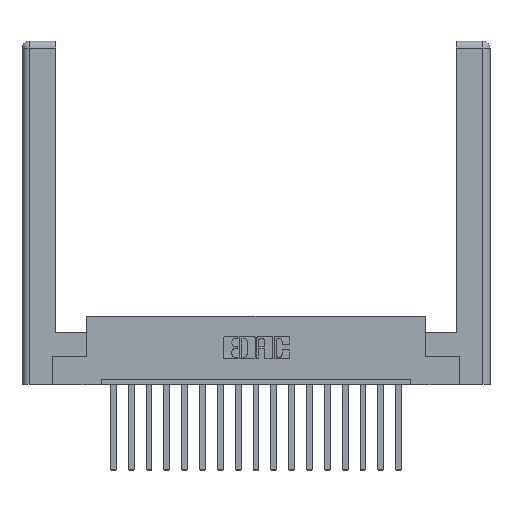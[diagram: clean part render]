
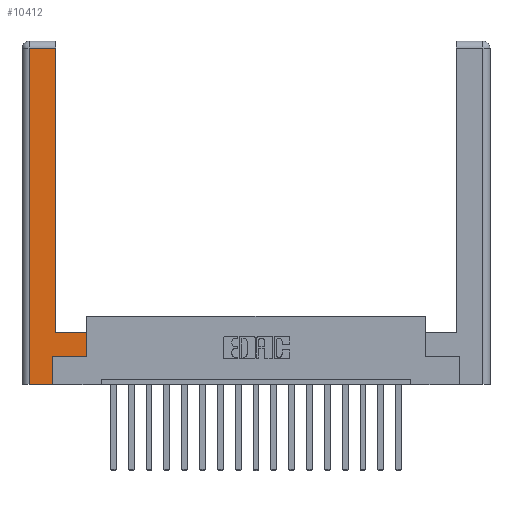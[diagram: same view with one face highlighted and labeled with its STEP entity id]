
A CAD part, top view. The second image highlights one B-rep face of the part: STEP entity #10412.
In plain terms, the highlighted planar face has unit normal (0, 0, 1).
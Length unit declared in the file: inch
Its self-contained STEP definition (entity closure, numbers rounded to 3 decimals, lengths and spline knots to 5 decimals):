
#91 = ORIENTED_EDGE ( 'NONE', *, *, #14278, .T. ) ;
#585 = VECTOR ( 'NONE', #4979, 39.37008 ) ;
#655 = CARTESIAN_POINT ( 'NONE',  ( 0.295, 0.45, 0. ) ) ;
#868 = VERTEX_POINT ( 'NONE', #13575 ) ;
#1252 = AXIS2_PLACEMENT_3D ( 'NONE', #9965, #9904, #9846 ) ;
#1298 = EDGE_CURVE ( 'NONE', #14913, #5578, #17673, .T. ) ;
#1403 = VECTOR ( 'NONE', #15407, 39.37008 ) ;
#1578 = CARTESIAN_POINT ( 'NONE',  ( 0.0615, 2.94, 0. ) ) ;
#1925 = VERTEX_POINT ( 'NONE', #12431 ) ;
#2137 = CARTESIAN_POINT ( 'NONE',  ( 0.0615, 2.94, 0. ) ) ;
#2154 = CARTESIAN_POINT ( 'NONE',  ( 0.565, 0.45, 0. ) ) ;
#2252 = ORIENTED_EDGE ( 'NONE', *, *, #13326, .T. ) ;
#2303 = DIRECTION ( 'NONE',  ( -1., 0., 0. ) ) ;
#2349 = VERTEX_POINT ( 'NONE', #655 ) ;
#2746 = DIRECTION ( 'NONE',  ( 1., 0., 0. ) ) ;
#3480 = VECTOR ( 'NONE', #2303, 39.37008 ) ;
#3620 = CARTESIAN_POINT ( 'NONE',  ( 0.0615, 0., 0. ) ) ;
#4251 = ORIENTED_EDGE ( 'NONE', *, *, #14342, .T. ) ;
#4393 = VECTOR ( 'NONE', #14295, 39.37008 ) ;
#4441 = EDGE_LOOP ( 'NONE', ( #16460, #12701, #6560, #2252, #91, #16508, #8641, #4251 ) ) ;
#4615 = LINE ( 'NONE', #1578, #4393 ) ;
#4620 = DIRECTION ( 'NONE',  ( 1., 0., 0. ) ) ;
#4720 = EDGE_CURVE ( 'NONE', #1925, #11762, #4615, .T. ) ;
#4979 = DIRECTION ( 'NONE',  ( 0., 1., 0. ) ) ;
#5578 = VERTEX_POINT ( 'NONE', #2154 ) ;
#5974 = CARTESIAN_POINT ( 'NONE',  ( 0.265, 0., 0. ) ) ;
#6349 = VERTEX_POINT ( 'NONE', #10061 ) ;
#6415 = VECTOR ( 'NONE', #16242, 39.37008 ) ;
#6509 = CARTESIAN_POINT ( 'NONE',  ( 0.295, 0.45, 0. ) ) ;
#6560 = ORIENTED_EDGE ( 'NONE', *, *, #11908, .T. ) ;
#6600 = EDGE_CURVE ( 'NONE', #2349, #1925, #16486, .T. ) ;
#6794 = LINE ( 'NONE', #13414, #585 ) ;
#6891 = CARTESIAN_POINT ( 'NONE',  ( 0.565, 0.245, 0. ) ) ;
#7680 = DIRECTION ( 'NONE',  ( 0., -1., 0. ) ) ;
#7972 = CARTESIAN_POINT ( 'NONE',  ( 0.565, 0.245, 0. ) ) ;
#8641 = ORIENTED_EDGE ( 'NONE', *, *, #1298, .T. ) ;
#8693 = PLANE ( 'NONE',  #1252 ) ;
#8758 = LINE ( 'NONE', #6509, #3480 ) ;
#8839 = VECTOR ( 'NONE', #7680, 39.37008 ) ;
#9343 = VERTEX_POINT ( 'NONE', #11339 ) ;
#9665 = VECTOR ( 'NONE', #2746, 39.37008 ) ;
#9846 = DIRECTION ( 'NONE',  ( -1., 0., 0. ) ) ;
#9904 = DIRECTION ( 'NONE',  ( 0., 0., -1. ) ) ;
#9965 = CARTESIAN_POINT ( 'NONE',  ( 0., 0., 0. ) ) ;
#10061 = CARTESIAN_POINT ( 'NONE',  ( 0.0615, 0., 0. ) ) ;
#10412 = ADVANCED_FACE ( 'NONE', ( #10854 ), #8693, .F. ) ;
#10854 = FACE_OUTER_BOUND ( 'NONE', #4441, .T. ) ;
#11169 = CARTESIAN_POINT ( 'NONE',  ( 0.295, 3., 0. ) ) ;
#11339 = CARTESIAN_POINT ( 'NONE',  ( 0.265, 0.245, 0. ) ) ;
#11762 = VERTEX_POINT ( 'NONE', #2137 ) ;
#11908 = EDGE_CURVE ( 'NONE', #11762, #6349, #16156, .T. ) ;
#12431 = CARTESIAN_POINT ( 'NONE',  ( 0.295, 2.94, 0. ) ) ;
#12701 = ORIENTED_EDGE ( 'NONE', *, *, #4720, .T. ) ;
#13185 = EDGE_CURVE ( 'NONE', #9343, #14913, #16769, .T. ) ;
#13326 = EDGE_CURVE ( 'NONE', #6349, #868, #14968, .T. ) ;
#13414 = CARTESIAN_POINT ( 'NONE',  ( 0.265, 0.245, 0. ) ) ;
#13575 = CARTESIAN_POINT ( 'NONE',  ( 0.265, 0., 0. ) ) ;
#14278 = EDGE_CURVE ( 'NONE', #868, #9343, #6794, .T. ) ;
#14295 = DIRECTION ( 'NONE',  ( -1., 0., 0. ) ) ;
#14342 = EDGE_CURVE ( 'NONE', #5578, #2349, #8758, .T. ) ;
#14913 = VERTEX_POINT ( 'NONE', #7972 ) ;
#14968 = LINE ( 'NONE', #5974, #18097 ) ;
#15407 = DIRECTION ( 'NONE',  ( 0., 1., 0. ) ) ;
#16156 = LINE ( 'NONE', #3620, #8839 ) ;
#16242 = DIRECTION ( 'NONE',  ( 0., 1., 0. ) ) ;
#16460 = ORIENTED_EDGE ( 'NONE', *, *, #6600, .T. ) ;
#16486 = LINE ( 'NONE', #11169, #1403 ) ;
#16508 = ORIENTED_EDGE ( 'NONE', *, *, #13185, .T. ) ;
#16769 = LINE ( 'NONE', #6891, #9665 ) ;
#17571 = CARTESIAN_POINT ( 'NONE',  ( 0.565, 0.45, 0. ) ) ;
#17673 = LINE ( 'NONE', #17571, #6415 ) ;
#18097 = VECTOR ( 'NONE', #4620, 39.37008 ) ;
